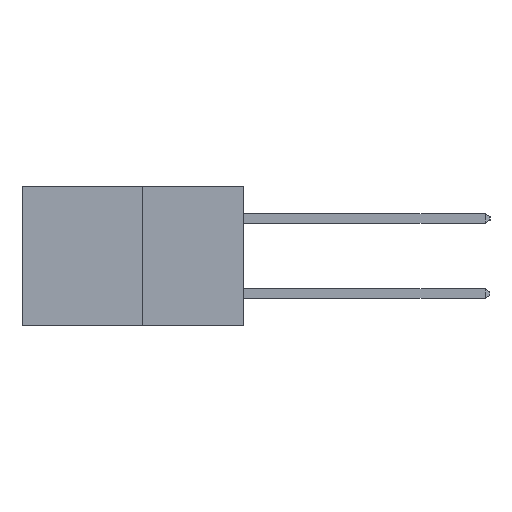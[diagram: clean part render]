
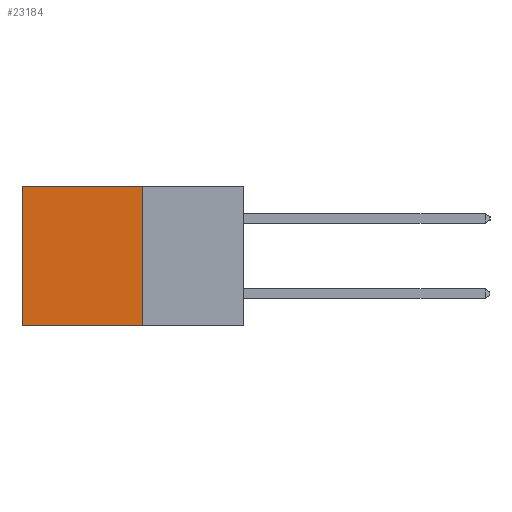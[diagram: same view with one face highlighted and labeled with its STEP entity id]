
A CAD part, left-side view. The second image highlights one B-rep face of the part: STEP entity #23184.
In plain terms, the highlighted planar face has unit normal (-1, 0, 0).
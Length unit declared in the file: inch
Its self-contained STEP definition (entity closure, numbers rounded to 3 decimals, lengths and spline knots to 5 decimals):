
#2717 = VECTOR ( 'NONE', #15659, 39.37008 ) ;
#2908 = VECTOR ( 'NONE', #21104, 39.37008 ) ;
#3243 = EDGE_LOOP ( 'NONE', ( #23023, #15695, #20639, #12664 ) ) ;
#3503 = LINE ( 'NONE', #8096, #2908 ) ;
#4513 = DIRECTION ( 'NONE',  ( 1., 0., 0. ) ) ;
#5143 = CARTESIAN_POINT ( 'NONE',  ( 0.277, 0.27, 0. ) ) ;
#6077 = CARTESIAN_POINT ( 'NONE',  ( 0.277, 0.27, -0.37 ) ) ;
#6351 = CARTESIAN_POINT ( 'NONE',  ( 0.277, 0.27, -0.37 ) ) ;
#6718 = EDGE_CURVE ( 'NONE', #9826, #15430, #14768, .T. ) ;
#7406 = VECTOR ( 'NONE', #23898, 39.37008 ) ;
#7478 = DIRECTION ( 'NONE',  ( 0., 1., 0. ) ) ;
#8096 = CARTESIAN_POINT ( 'NONE',  ( 0.277, 0.59, -0.37 ) ) ;
#8212 = EDGE_CURVE ( 'NONE', #9826, #22361, #22236, .T. ) ;
#9116 = AXIS2_PLACEMENT_3D ( 'NONE', #15777, #4513, #17614 ) ;
#9826 = VERTEX_POINT ( 'NONE', #11141 ) ;
#10753 = EDGE_CURVE ( 'NONE', #15430, #14708, #3503, .T. ) ;
#11141 = CARTESIAN_POINT ( 'NONE',  ( 0.277, 0.27, 0. ) ) ;
#12664 = ORIENTED_EDGE ( 'NONE', *, *, #6718, .T. ) ;
#13917 = PLANE ( 'NONE',  #9116 ) ;
#14215 = LINE ( 'NONE', #6351, #2717 ) ;
#14708 = VERTEX_POINT ( 'NONE', #14942 ) ;
#14768 = LINE ( 'NONE', #5143, #19082 ) ;
#14942 = CARTESIAN_POINT ( 'NONE',  ( 0.277, 0.59, -0.37 ) ) ;
#15001 = EDGE_CURVE ( 'NONE', #22361, #14708, #14215, .T. ) ;
#15430 = VERTEX_POINT ( 'NONE', #21980 ) ;
#15659 = DIRECTION ( 'NONE',  ( 0., 1., 0. ) ) ;
#15695 = ORIENTED_EDGE ( 'NONE', *, *, #15001, .F. ) ;
#15777 = CARTESIAN_POINT ( 'NONE',  ( 0.277, 0.27, -0.37 ) ) ;
#17614 = DIRECTION ( 'NONE',  ( 0., 0., -1. ) ) ;
#19082 = VECTOR ( 'NONE', #7478, 39.37008 ) ;
#20639 = ORIENTED_EDGE ( 'NONE', *, *, #8212, .F. ) ;
#21104 = DIRECTION ( 'NONE',  ( 0., 0., -1. ) ) ;
#21980 = CARTESIAN_POINT ( 'NONE',  ( 0.277, 0.59, 0. ) ) ;
#22236 = LINE ( 'NONE', #24020, #7406 ) ;
#22361 = VERTEX_POINT ( 'NONE', #6077 ) ;
#23023 = ORIENTED_EDGE ( 'NONE', *, *, #10753, .T. ) ;
#23184 = ADVANCED_FACE ( 'NONE', ( #24326 ), #13917, .F. ) ;
#23898 = DIRECTION ( 'NONE',  ( 0., 0., -1. ) ) ;
#24020 = CARTESIAN_POINT ( 'NONE',  ( 0.277, 0.27, -0.37 ) ) ;
#24326 = FACE_OUTER_BOUND ( 'NONE', #3243, .T. ) ;
